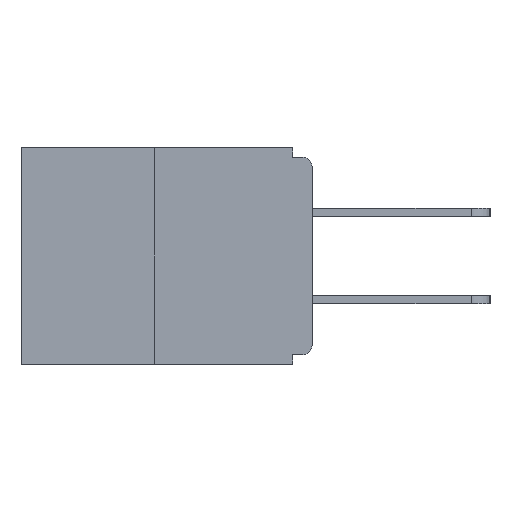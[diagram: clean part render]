
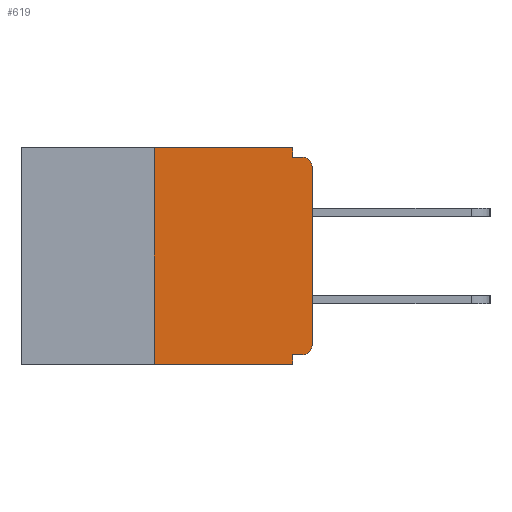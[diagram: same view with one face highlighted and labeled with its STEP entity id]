
A CAD part, left-side view. The second image highlights one B-rep face of the part: STEP entity #619.
In plain terms, the highlighted planar face has unit normal (-1, 0, 0).
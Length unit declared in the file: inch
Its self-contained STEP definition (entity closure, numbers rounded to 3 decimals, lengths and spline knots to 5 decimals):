
#263 = EDGE_CURVE ( 'NONE', #19420, #19199, #4443, .T. ) ;
#310 = CARTESIAN_POINT ( 'NONE',  ( 0., 0.25, 0. ) ) ;
#523 = LINE ( 'NONE', #8902, #7514 ) ;
#619 = ADVANCED_FACE ( 'NONE', ( #1158 ), #17806, .F. ) ;
#823 = CARTESIAN_POINT ( 'NONE',  ( 0., 0., -0.328 ) ) ;
#1158 = FACE_OUTER_BOUND ( 'NONE', #23427, .T. ) ;
#1406 = CARTESIAN_POINT ( 'NONE',  ( 0., 0.25, -0.343 ) ) ;
#1482 = ORIENTED_EDGE ( 'NONE', *, *, #4497, .T. ) ;
#1607 = LINE ( 'NONE', #10764, #15767 ) ;
#1678 = CARTESIAN_POINT ( 'NONE',  ( 0., 0.46, -0.343 ) ) ;
#2621 = DIRECTION ( 'NONE',  ( 0., 0., -1. ) ) ;
#3697 = EDGE_CURVE ( 'NONE', #21400, #12816, #23096, .T. ) ;
#3756 = VERTEX_POINT ( 'NONE', #19979 ) ;
#3758 = ORIENTED_EDGE ( 'NONE', *, *, #17517, .F. ) ;
#4347 = DIRECTION ( 'NONE',  ( -1., 0., 0. ) ) ;
#4443 = LINE ( 'NONE', #10116, #18196 ) ;
#4497 = EDGE_CURVE ( 'NONE', #15819, #12816, #16053, .T. ) ;
#4542 = ORIENTED_EDGE ( 'NONE', *, *, #3697, .F. ) ;
#4817 = CARTESIAN_POINT ( 'NONE',  ( 0., 0.46, 0. ) ) ;
#4868 = DIRECTION ( 'NONE',  ( 1., 0., 0. ) ) ;
#4904 = LINE ( 'NONE', #823, #5432 ) ;
#5432 = VECTOR ( 'NONE', #10108, 39.37008 ) ;
#6680 = DIRECTION ( 'NONE',  ( 0., 0., -1. ) ) ;
#7150 = ORIENTED_EDGE ( 'NONE', *, *, #20744, .T. ) ;
#7514 = VECTOR ( 'NONE', #20003, 39.37008 ) ;
#7794 = VERTEX_POINT ( 'NONE', #9226 ) ;
#8735 = CARTESIAN_POINT ( 'NONE',  ( 0., 0.46, 0. ) ) ;
#8902 = CARTESIAN_POINT ( 'NONE',  ( 0., 0.031, -0.343 ) ) ;
#9131 = AXIS2_PLACEMENT_3D ( 'NONE', #22814, #4347, #19204 ) ;
#9226 = CARTESIAN_POINT ( 'NONE',  ( 0., 0.031, -0.343 ) ) ;
#9986 = DIRECTION ( 'NONE',  ( 0., 0., 1. ) ) ;
#10108 = DIRECTION ( 'NONE',  ( 0., 1., 0. ) ) ;
#10116 = CARTESIAN_POINT ( 'NONE',  ( 0., 0.25, 0. ) ) ;
#10421 = VECTOR ( 'NONE', #14544, 39.37008 ) ;
#10506 = LINE ( 'NONE', #4817, #12526 ) ;
#10764 = CARTESIAN_POINT ( 'NONE',  ( 0., 0., 0. ) ) ;
#10765 = CARTESIAN_POINT ( 'NONE',  ( 0., 0.031, 0. ) ) ;
#10869 = ORIENTED_EDGE ( 'NONE', *, *, #21581, .F. ) ;
#12066 = ORIENTED_EDGE ( 'NONE', *, *, #13039, .T. ) ;
#12526 = VECTOR ( 'NONE', #17868, 39.37008 ) ;
#12816 = VERTEX_POINT ( 'NONE', #23376 ) ;
#12896 = CARTESIAN_POINT ( 'NONE',  ( 0., 0., -0.03 ) ) ;
#13039 = EDGE_CURVE ( 'NONE', #22435, #21813, #16241, .T. ) ;
#13240 = DIRECTION ( 'NONE',  ( -1., 0., 0. ) ) ;
#13736 = VECTOR ( 'NONE', #19262, 39.37008 ) ;
#13830 = VERTEX_POINT ( 'NONE', #10765 ) ;
#14014 = ORIENTED_EDGE ( 'NONE', *, *, #18973, .T. ) ;
#14193 = CARTESIAN_POINT ( 'NONE',  ( 0., 0., -0.015 ) ) ;
#14210 = ORIENTED_EDGE ( 'NONE', *, *, #263, .F. ) ;
#14320 = AXIS2_PLACEMENT_3D ( 'NONE', #15055, #13240, #2621 ) ;
#14544 = DIRECTION ( 'NONE',  ( 0., 0., -1. ) ) ;
#14811 = LINE ( 'NONE', #1678, #15356 ) ;
#15055 = CARTESIAN_POINT ( 'NONE',  ( 0., 0.015, -0.313 ) ) ;
#15356 = VECTOR ( 'NONE', #16499, 39.37008 ) ;
#15767 = VECTOR ( 'NONE', #18141, 39.37008 ) ;
#15819 = VERTEX_POINT ( 'NONE', #12896 ) ;
#15934 = ORIENTED_EDGE ( 'NONE', *, *, #23466, .F. ) ;
#15964 = ORIENTED_EDGE ( 'NONE', *, *, #18447, .F. ) ;
#16053 = CIRCLE ( 'NONE', #9131, 0.015 ) ;
#16241 = CIRCLE ( 'NONE', #14320, 0.015 ) ;
#16499 = DIRECTION ( 'NONE',  ( 0., -1., 0. ) ) ;
#17056 = CARTESIAN_POINT ( 'NONE',  ( 0., 0.015, -0.328 ) ) ;
#17517 = EDGE_CURVE ( 'NONE', #3756, #7794, #523, .T. ) ;
#17806 = PLANE ( 'NONE',  #18605 ) ;
#17868 = DIRECTION ( 'NONE',  ( 0., -1., 0. ) ) ;
#18141 = DIRECTION ( 'NONE',  ( 0., 0., 1. ) ) ;
#18179 = CARTESIAN_POINT ( 'NONE',  ( 0., 0.031, 0. ) ) ;
#18196 = VECTOR ( 'NONE', #9986, 39.37008 ) ;
#18447 = EDGE_CURVE ( 'NONE', #19199, #13830, #10506, .T. ) ;
#18605 = AXIS2_PLACEMENT_3D ( 'NONE', #8735, #4868, #6680 ) ;
#18973 = EDGE_CURVE ( 'NONE', #19420, #7794, #14811, .T. ) ;
#19199 = VERTEX_POINT ( 'NONE', #310 ) ;
#19204 = DIRECTION ( 'NONE',  ( 0., 0., -1. ) ) ;
#19262 = DIRECTION ( 'NONE',  ( 0., -1., 0. ) ) ;
#19420 = VERTEX_POINT ( 'NONE', #1406 ) ;
#19979 = CARTESIAN_POINT ( 'NONE',  ( 0., 0.031, -0.328 ) ) ;
#20003 = DIRECTION ( 'NONE',  ( 0., 0., -1. ) ) ;
#20744 = EDGE_CURVE ( 'NONE', #21813, #15819, #1607, .T. ) ;
#21283 = LINE ( 'NONE', #18179, #10421 ) ;
#21400 = VERTEX_POINT ( 'NONE', #22964 ) ;
#21581 = EDGE_CURVE ( 'NONE', #13830, #21400, #21283, .T. ) ;
#21813 = VERTEX_POINT ( 'NONE', #22941 ) ;
#22435 = VERTEX_POINT ( 'NONE', #17056 ) ;
#22814 = CARTESIAN_POINT ( 'NONE',  ( 0., 0.015, -0.03 ) ) ;
#22941 = CARTESIAN_POINT ( 'NONE',  ( 0., 0., -0.313 ) ) ;
#22964 = CARTESIAN_POINT ( 'NONE',  ( 0., 0.031, -0.015 ) ) ;
#23096 = LINE ( 'NONE', #14193, #13736 ) ;
#23376 = CARTESIAN_POINT ( 'NONE',  ( 0., 0.015, -0.015 ) ) ;
#23427 = EDGE_LOOP ( 'NONE', ( #15964, #14210, #14014, #3758, #15934, #12066, #7150, #1482, #4542, #10869 ) ) ;
#23466 = EDGE_CURVE ( 'NONE', #22435, #3756, #4904, .T. ) ;
